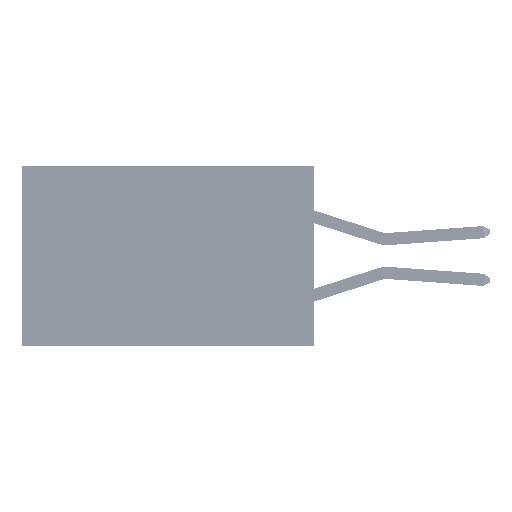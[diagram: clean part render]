
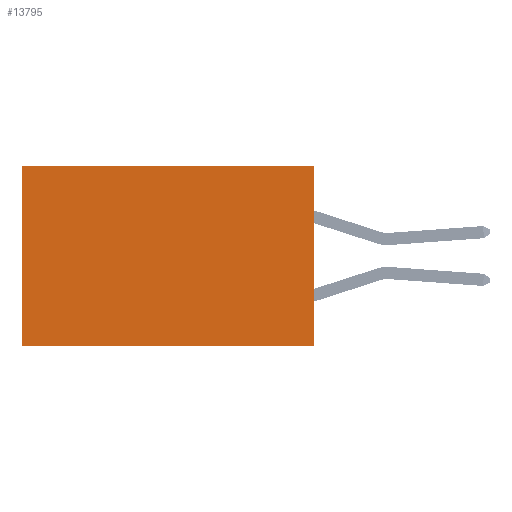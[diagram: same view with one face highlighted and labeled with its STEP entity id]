
A CAD part, left-side view. The second image highlights one B-rep face of the part: STEP entity #13795.
In plain terms, the highlighted planar face has unit normal (-1, 0, 0).
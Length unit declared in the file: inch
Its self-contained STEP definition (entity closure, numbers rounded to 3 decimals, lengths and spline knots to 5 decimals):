
#2498 = VERTEX_POINT ( 'NONE', #28612 ) ;
#3162 = EDGE_CURVE ( 'NONE', #22729, #2498, #35182, .T. ) ;
#3598 = CARTESIAN_POINT ( 'NONE',  ( 0.2875, 0., 0. ) ) ;
#5037 = VECTOR ( 'NONE', #21353, 39.37008 ) ;
#10065 = DIRECTION ( 'NONE',  ( 1., 0., 0. ) ) ;
#13795 = ADVANCED_FACE ( 'NONE', ( #24201 ), #28566, .F. ) ;
#15849 = CARTESIAN_POINT ( 'NONE',  ( 0.2875, 0.6, -0.37 ) ) ;
#16649 = CARTESIAN_POINT ( 'NONE',  ( 0.2875, 0., 0. ) ) ;
#16708 = LINE ( 'NONE', #16649, #27827 ) ;
#17268 = CARTESIAN_POINT ( 'NONE',  ( 0.2875, 0.6, 0. ) ) ;
#18011 = EDGE_CURVE ( 'NONE', #2498, #39763, #44164, .T. ) ;
#18327 = VECTOR ( 'NONE', #42109, 39.37008 ) ;
#19470 = DIRECTION ( 'NONE',  ( 0., 1., 0. ) ) ;
#20191 = ORIENTED_EDGE ( 'NONE', *, *, #3162, .T. ) ;
#20492 = CARTESIAN_POINT ( 'NONE',  ( 0.2875, 0., 0. ) ) ;
#20833 = CARTESIAN_POINT ( 'NONE',  ( 0.2875, 0., -0.37 ) ) ;
#21332 = ORIENTED_EDGE ( 'NONE', *, *, #30857, .F. ) ;
#21353 = DIRECTION ( 'NONE',  ( 0., 0., -1. ) ) ;
#22729 = VERTEX_POINT ( 'NONE', #20492 ) ;
#24201 = FACE_OUTER_BOUND ( 'NONE', #41271, .T. ) ;
#25119 = DIRECTION ( 'NONE',  ( 0., 0., -1. ) ) ;
#27827 = VECTOR ( 'NONE', #42647, 39.37008 ) ;
#28566 = PLANE ( 'NONE',  #41347 ) ;
#28612 = CARTESIAN_POINT ( 'NONE',  ( 0.2875, 0.6, 0. ) ) ;
#28890 = ORIENTED_EDGE ( 'NONE', *, *, #18011, .T. ) ;
#30668 = LINE ( 'NONE', #42595, #18327 ) ;
#30857 = EDGE_CURVE ( 'NONE', #40862, #39763, #30668, .T. ) ;
#32472 = CARTESIAN_POINT ( 'NONE',  ( 0.2875, 0., 0. ) ) ;
#32578 = ORIENTED_EDGE ( 'NONE', *, *, #43669, .F. ) ;
#35182 = LINE ( 'NONE', #3598, #36902 ) ;
#36902 = VECTOR ( 'NONE', #19470, 39.37008 ) ;
#39763 = VERTEX_POINT ( 'NONE', #15849 ) ;
#40862 = VERTEX_POINT ( 'NONE', #20833 ) ;
#41271 = EDGE_LOOP ( 'NONE', ( #28890, #21332, #32578, #20191 ) ) ;
#41347 = AXIS2_PLACEMENT_3D ( 'NONE', #32472, #10065, #25119 ) ;
#42109 = DIRECTION ( 'NONE',  ( 0., 1., 0. ) ) ;
#42595 = CARTESIAN_POINT ( 'NONE',  ( 0.2875, 0., -0.37 ) ) ;
#42647 = DIRECTION ( 'NONE',  ( 0., 0., -1. ) ) ;
#43669 = EDGE_CURVE ( 'NONE', #22729, #40862, #16708, .T. ) ;
#44164 = LINE ( 'NONE', #17268, #5037 ) ;
